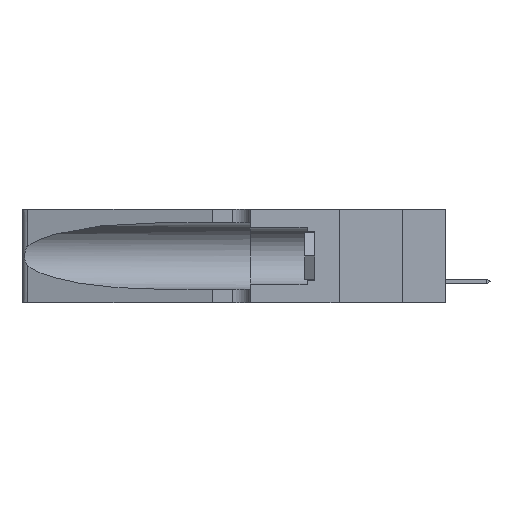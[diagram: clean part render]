
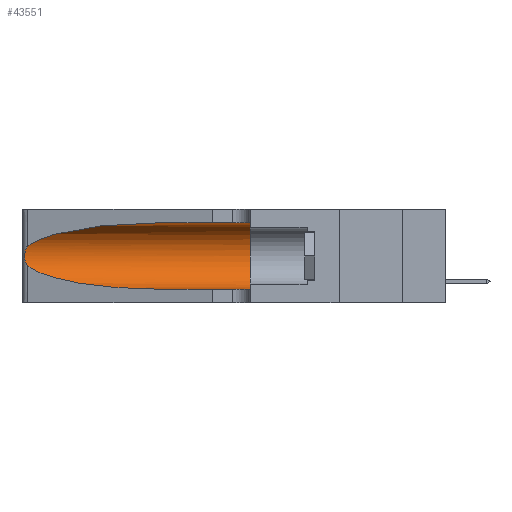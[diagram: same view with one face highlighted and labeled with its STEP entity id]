
A CAD part, left-side view. The second image highlights one B-rep face of the part: STEP entity #43551.
In plain terms, the highlighted cylindrical face has radius 3.308 mm (diameter 6.617 mm), a partial arc.
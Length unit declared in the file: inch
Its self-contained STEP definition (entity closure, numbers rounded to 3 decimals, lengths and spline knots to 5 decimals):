
#176 = DIRECTION ( 'NONE',  ( 0., 0., 1. ) ) ;
#664 = EDGE_CURVE ( 'NONE', #32952, #37755, #42535, .T. ) ;
#906 = ORIENTED_EDGE ( 'NONE', *, *, #9352, .T. ) ;
#1649 = CARTESIAN_POINT ( 'NONE',  ( 0.1305, 0.72297, 0.31525 ) ) ;
#2187 = EDGE_CURVE ( 'NONE', #17057, #32952, #35799, .T. ) ;
#2486 = CARTESIAN_POINT ( 'NONE',  ( 0.1305, 0.35, 0.31525 ) ) ;
#3037 = EDGE_CURVE ( 'NONE', #40941, #37755, #39886, .T. ) ;
#4191 = B_SPLINE_CURVE_WITH_KNOTS ( 'NONE', 3,
 ( #21833, #15187, #8891, #39538, #32606, #25769, #5480, #18591, #19166, #11882, #35557, #35871, #5002, #42746 ),
 .UNSPECIFIED., .F., .F.,
 ( 4, 2, 2, 2, 2, 2, 4 ),
 ( 0., 0.00027, 0.00053, 0.00107, 0.0016, 0.00187, 0.00214 ),
 .UNSPECIFIED. ) ;
#4847 = CARTESIAN_POINT ( 'NONE',  ( 0.1305, 0.72297, 0.05475 ) ) ;
#5002 = CARTESIAN_POINT ( 'NONE',  ( 0.25555, 1.22993, 0.14849 ) ) ;
#5480 = CARTESIAN_POINT ( 'NONE',  ( 0.26075, 1.23896, 0.19203 ) ) ;
#5979 = CARTESIAN_POINT ( 'NONE',  ( 0.25487, 1.22718, 0.14631 ) ) ;
#6255 = VECTOR ( 'NONE', #22743, 39.37008 ) ;
#8537 = EDGE_CURVE ( 'NONE', #32826, #17057, #4191, .T. ) ;
#8891 = CARTESIAN_POINT ( 'NONE',  ( 0.25639, 1.23184, 0.21858 ) ) ;
#9019 = CARTESIAN_POINT ( 'NONE',  ( 0.2373, 1.15595, 0.28018 ) ) ;
#9352 = EDGE_CURVE ( 'NONE', #29870, #32826, #10273, .T. ) ;
#10273 =( BOUNDED_CURVE ( )  B_SPLINE_CURVE ( 3, ( #1649, #28849, #9019, #32120 ),
 .UNSPECIFIED., .F., .F. ) 
 B_SPLINE_CURVE_WITH_KNOTS ( ( 4, 4 ),
 ( 1.5708, 2.84003 ),
 .UNSPECIFIED. ) 
 CURVE ( )  GEOMETRIC_REPRESENTATION_ITEM ( )  RATIONAL_B_SPLINE_CURVE ( ( 1., 0.87, 0.87, 1. ) ) 
 REPRESENTATION_ITEM ( '' )  );
#10277 = VECTOR ( 'NONE', #15159, 39.37008 ) ;
#10668 = CARTESIAN_POINT ( 'NONE',  ( 0.18966, 0.96281, 0.05475 ) ) ;
#11216 = ORIENTED_EDGE ( 'NONE', *, *, #664, .T. ) ;
#11664 = AXIS2_PLACEMENT_3D ( 'NONE', #40822, #24376, #27957 ) ;
#11822 = AXIS2_PLACEMENT_3D ( 'NONE', #17269, #20521, #176 ) ;
#11882 = CARTESIAN_POINT ( 'NONE',  ( 0.25856, 1.23593, 0.16098 ) ) ;
#12897 = CARTESIAN_POINT ( 'NONE',  ( 0.25487, 1.22718, 0.22369 ) ) ;
#15159 = DIRECTION ( 'NONE',  ( 0., -1., 0. ) ) ;
#15187 = CARTESIAN_POINT ( 'NONE',  ( 0.25555, 1.22994, 0.2215 ) ) ;
#17057 = VERTEX_POINT ( 'NONE', #5979 ) ;
#17128 = ORIENTED_EDGE ( 'NONE', *, *, #2187, .T. ) ;
#17269 = CARTESIAN_POINT ( 'NONE',  ( 0.1305, 0.35, 0.185 ) ) ;
#18591 = CARTESIAN_POINT ( 'NONE',  ( 0.26075, 1.23896, 0.178 ) ) ;
#19166 = CARTESIAN_POINT ( 'NONE',  ( 0.26017, 1.23833, 0.17102 ) ) ;
#20521 = DIRECTION ( 'NONE',  ( 0., 1., 0. ) ) ;
#21641 = CYLINDRICAL_SURFACE ( 'NONE', #11664, 0.13025 ) ;
#21833 = CARTESIAN_POINT ( 'NONE',  ( 0.25487, 1.22718, 0.22369 ) ) ;
#22446 = CARTESIAN_POINT ( 'NONE',  ( 0.1305, 1.61858, 0.05475 ) ) ;
#22743 = DIRECTION ( 'NONE',  ( 0., -1., 0. ) ) ;
#24232 = CARTESIAN_POINT ( 'NONE',  ( 0.1305, 0.72297, 0.05475 ) ) ;
#24376 = DIRECTION ( 'NONE',  ( 0., -1., 0. ) ) ;
#24387 = EDGE_CURVE ( 'NONE', #29870, #40941, #24740, .T. ) ;
#24554 = EDGE_LOOP ( 'NONE', ( #906, #42330, #17128, #11216, #28314, #35492 ) ) ;
#24740 = LINE ( 'NONE', #30046, #6255 ) ;
#25769 = CARTESIAN_POINT ( 'NONE',  ( 0.26018, 1.23835, 0.19895 ) ) ;
#27957 = DIRECTION ( 'NONE',  ( 0., 0., -1. ) ) ;
#28314 = ORIENTED_EDGE ( 'NONE', *, *, #3037, .F. ) ;
#28849 = CARTESIAN_POINT ( 'NONE',  ( 0.18966, 0.96281, 0.31525 ) ) ;
#29162 = FACE_OUTER_BOUND ( 'NONE', #24554, .T. ) ;
#29870 = VERTEX_POINT ( 'NONE', #41451 ) ;
#30046 = CARTESIAN_POINT ( 'NONE',  ( 0.1305, 1.61858, 0.31525 ) ) ;
#32120 = CARTESIAN_POINT ( 'NONE',  ( 0.25487, 1.22718, 0.22369 ) ) ;
#32606 = CARTESIAN_POINT ( 'NONE',  ( 0.25854, 1.2359, 0.20912 ) ) ;
#32826 = VERTEX_POINT ( 'NONE', #12897 ) ;
#32952 = VERTEX_POINT ( 'NONE', #4847 ) ;
#34211 = CARTESIAN_POINT ( 'NONE',  ( 0.2373, 1.15595, 0.08982 ) ) ;
#35492 = ORIENTED_EDGE ( 'NONE', *, *, #24387, .F. ) ;
#35557 = CARTESIAN_POINT ( 'NONE',  ( 0.25789, 1.23486, 0.15765 ) ) ;
#35799 =( BOUNDED_CURVE ( )  B_SPLINE_CURVE ( 3, ( #40948, #34211, #10668, #24232 ),
 .UNSPECIFIED., .F., .T. ) 
 B_SPLINE_CURVE_WITH_KNOTS ( ( 4, 4 ),
 ( 3.44316, 4.71239 ),
 .UNSPECIFIED. ) 
 CURVE ( )  GEOMETRIC_REPRESENTATION_ITEM ( )  RATIONAL_B_SPLINE_CURVE ( ( 1., 0.87, 0.87, 1. ) ) 
 REPRESENTATION_ITEM ( '' )  );
#35871 = CARTESIAN_POINT ( 'NONE',  ( 0.25639, 1.23186, 0.15144 ) ) ;
#37755 = VERTEX_POINT ( 'NONE', #39577 ) ;
#39538 = CARTESIAN_POINT ( 'NONE',  ( 0.25787, 1.23484, 0.2124 ) ) ;
#39577 = CARTESIAN_POINT ( 'NONE',  ( 0.1305, 0.35, 0.05475 ) ) ;
#39886 = CIRCLE ( 'NONE', #11822, 0.13025 ) ;
#40822 = CARTESIAN_POINT ( 'NONE',  ( 0.1305, 1.61858, 0.185 ) ) ;
#40941 = VERTEX_POINT ( 'NONE', #2486 ) ;
#40948 = CARTESIAN_POINT ( 'NONE',  ( 0.25487, 1.22718, 0.14631 ) ) ;
#41451 = CARTESIAN_POINT ( 'NONE',  ( 0.1305, 0.72297, 0.31525 ) ) ;
#42330 = ORIENTED_EDGE ( 'NONE', *, *, #8537, .T. ) ;
#42535 = LINE ( 'NONE', #22446, #10277 ) ;
#42746 = CARTESIAN_POINT ( 'NONE',  ( 0.25487, 1.22718, 0.14631 ) ) ;
#43551 = ADVANCED_FACE ( 'NONE', ( #29162 ), #21641, .F. ) ;
